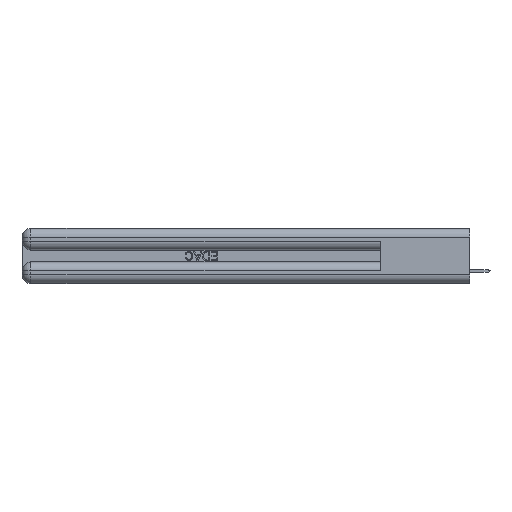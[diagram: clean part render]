
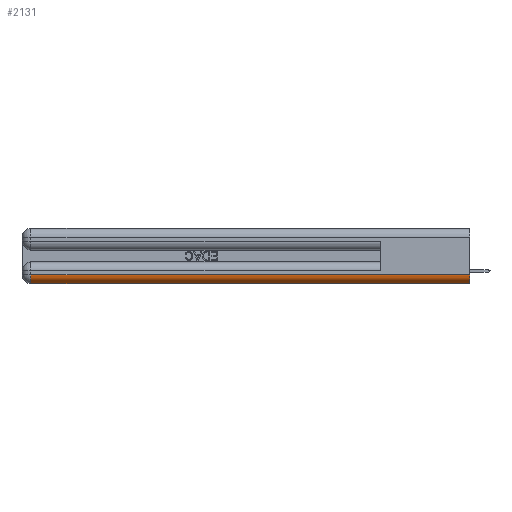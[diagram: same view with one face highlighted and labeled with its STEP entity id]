
A CAD part, left-side view. The second image highlights one B-rep face of the part: STEP entity #2131.
In plain terms, the highlighted cylindrical face has radius 1.524 mm (diameter 3.048 mm), a partial arc.
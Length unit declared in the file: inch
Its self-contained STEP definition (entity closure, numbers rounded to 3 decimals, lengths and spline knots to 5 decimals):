
#308 = DIRECTION ( 'NONE',  ( 0., 0., 1. ) ) ;
#330 = LINE ( 'NONE', #12456, #20540 ) ;
#686 = VERTEX_POINT ( 'NONE', #13590 ) ;
#909 = DIRECTION ( 'NONE',  ( 0., 1., 0. ) ) ;
#1498 = DIRECTION ( 'NONE',  ( 0., 1., 0. ) ) ;
#1623 = VERTEX_POINT ( 'NONE', #28473 ) ;
#2131 = ADVANCED_FACE ( 'NONE', ( #12703 ), #12904, .T. ) ;
#2507 = CARTESIAN_POINT ( 'NONE',  ( 0.06, 0., 0.06 ) ) ;
#2747 = VERTEX_POINT ( 'NONE', #26190 ) ;
#3826 = VECTOR ( 'NONE', #32943, 39.37008 ) ;
#3872 = CARTESIAN_POINT ( 'NONE',  ( 0.06, 2.94, 0.06 ) ) ;
#3929 = DIRECTION ( 'NONE',  ( 0., 1., 0. ) ) ;
#6023 = LINE ( 'NONE', #30177, #3826 ) ;
#6649 = ORIENTED_EDGE ( 'NONE', *, *, #9511, .F. ) ;
#9511 = EDGE_CURVE ( 'NONE', #1623, #2747, #34925, .T. ) ;
#9799 = CARTESIAN_POINT ( 'NONE',  ( 0., 0., 0.06 ) ) ;
#12456 = CARTESIAN_POINT ( 'NONE',  ( 0.06, 3., 0. ) ) ;
#12460 = EDGE_CURVE ( 'NONE', #2747, #12643, #6023, .T. ) ;
#12643 = VERTEX_POINT ( 'NONE', #9799 ) ;
#12703 = FACE_OUTER_BOUND ( 'NONE', #19929, .T. ) ;
#12904 = CYLINDRICAL_SURFACE ( 'NONE', #22503, 0.06 ) ;
#13290 = ORIENTED_EDGE ( 'NONE', *, *, #18109, .F. ) ;
#13532 = ORIENTED_EDGE ( 'NONE', *, *, #12460, .F. ) ;
#13590 = CARTESIAN_POINT ( 'NONE',  ( 0.06, 0., 0. ) ) ;
#14086 = EDGE_CURVE ( 'NONE', #686, #1623, #330, .T. ) ;
#18109 = EDGE_CURVE ( 'NONE', #12643, #686, #21035, .T. ) ;
#19455 = CARTESIAN_POINT ( 'NONE',  ( 0.06, 0., 0.06 ) ) ;
#19929 = EDGE_LOOP ( 'NONE', ( #13290, #13532, #6649, #22494 ) ) ;
#20540 = VECTOR ( 'NONE', #909, 39.37008 ) ;
#21035 = CIRCLE ( 'NONE', #28017, 0.06 ) ;
#22494 = ORIENTED_EDGE ( 'NONE', *, *, #14086, .F. ) ;
#22503 = AXIS2_PLACEMENT_3D ( 'NONE', #19455, #3929, #34610 ) ;
#22843 = AXIS2_PLACEMENT_3D ( 'NONE', #3872, #1498, #28956 ) ;
#26190 = CARTESIAN_POINT ( 'NONE',  ( 0., 2.94, 0.06 ) ) ;
#26807 = DIRECTION ( 'NONE',  ( 0., -1., 0. ) ) ;
#28017 = AXIS2_PLACEMENT_3D ( 'NONE', #2507, #26807, #308 ) ;
#28473 = CARTESIAN_POINT ( 'NONE',  ( 0.06, 2.94, 0. ) ) ;
#28956 = DIRECTION ( 'NONE',  ( 0., 0., 1. ) ) ;
#30177 = CARTESIAN_POINT ( 'NONE',  ( 0., 0., 0.06 ) ) ;
#32943 = DIRECTION ( 'NONE',  ( 0., -1., 0. ) ) ;
#34610 = DIRECTION ( 'NONE',  ( 0., 0., 1. ) ) ;
#34925 = CIRCLE ( 'NONE', #22843, 0.06 ) ;
